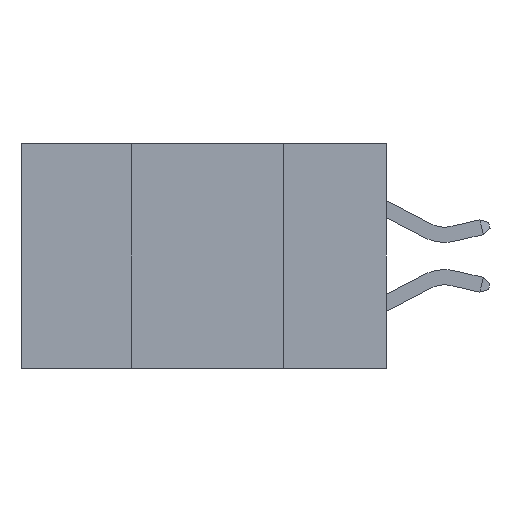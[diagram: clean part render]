
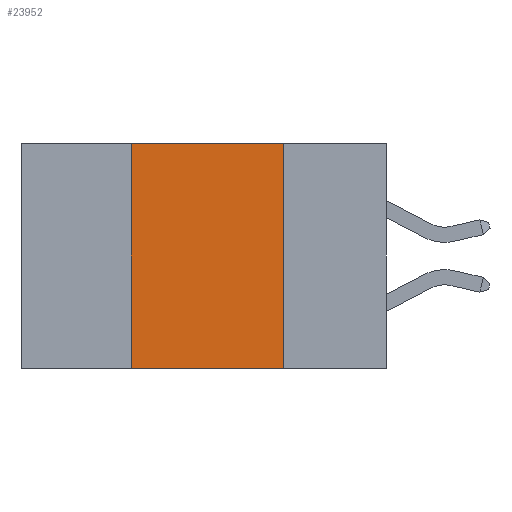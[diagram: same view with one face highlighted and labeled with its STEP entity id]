
A CAD part, left-side view. The second image highlights one B-rep face of the part: STEP entity #23952.
In plain terms, the highlighted planar face has unit normal (-1, 0, 0).
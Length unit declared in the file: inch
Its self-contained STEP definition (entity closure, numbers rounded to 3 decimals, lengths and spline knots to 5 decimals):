
#594 = LINE ( 'NONE', #15089, #6011 ) ;
#796 = VECTOR ( 'NONE', #20735, 39.37008 ) ;
#1096 = FACE_OUTER_BOUND ( 'NONE', #6258, .T. ) ;
#1642 = VERTEX_POINT ( 'NONE', #17662 ) ;
#1765 = EDGE_CURVE ( 'NONE', #1642, #24091, #3038, .T. ) ;
#2606 = EDGE_CURVE ( 'NONE', #1642, #14777, #594, .T. ) ;
#2847 = VECTOR ( 'NONE', #5439, 39.37008 ) ;
#3038 = LINE ( 'NONE', #17379, #25171 ) ;
#5439 = DIRECTION ( 'NONE',  ( 0., -1., 0. ) ) ;
#6011 = VECTOR ( 'NONE', #6787, 39.37008 ) ;
#6258 = EDGE_LOOP ( 'NONE', ( #8820, #11707, #11270, #15451 ) ) ;
#6787 = DIRECTION ( 'NONE',  ( 0., 0., 1. ) ) ;
#8058 = AXIS2_PLACEMENT_3D ( 'NONE', #13023, #9272, #19251 ) ;
#8820 = ORIENTED_EDGE ( 'NONE', *, *, #14018, .F. ) ;
#9272 = DIRECTION ( 'NONE',  ( 1., 0., 0. ) ) ;
#11270 = ORIENTED_EDGE ( 'NONE', *, *, #2606, .F. ) ;
#11707 = ORIENTED_EDGE ( 'NONE', *, *, #21804, .F. ) ;
#12501 = LINE ( 'NONE', #16564, #796 ) ;
#13023 = CARTESIAN_POINT ( 'NONE',  ( 0., 0.6, 0. ) ) ;
#14018 = EDGE_CURVE ( 'NONE', #20674, #24091, #12501, .T. ) ;
#14777 = VERTEX_POINT ( 'NONE', #15991 ) ;
#14785 = PLANE ( 'NONE',  #8058 ) ;
#15089 = CARTESIAN_POINT ( 'NONE',  ( 0., 0.42, -0.37 ) ) ;
#15451 = ORIENTED_EDGE ( 'NONE', *, *, #1765, .T. ) ;
#15886 = CARTESIAN_POINT ( 'NONE',  ( 0., 0.17, -0.37 ) ) ;
#15991 = CARTESIAN_POINT ( 'NONE',  ( 0., 0.42, 0. ) ) ;
#16320 = CARTESIAN_POINT ( 'NONE',  ( 0., 0.17, 0. ) ) ;
#16564 = CARTESIAN_POINT ( 'NONE',  ( 0., 0.17, -0.37 ) ) ;
#17379 = CARTESIAN_POINT ( 'NONE',  ( 0., 0.6, -0.37 ) ) ;
#17662 = CARTESIAN_POINT ( 'NONE',  ( 0., 0.42, -0.37 ) ) ;
#18285 = LINE ( 'NONE', #23865, #2847 ) ;
#19251 = DIRECTION ( 'NONE',  ( 0., 0., -1. ) ) ;
#20674 = VERTEX_POINT ( 'NONE', #16320 ) ;
#20735 = DIRECTION ( 'NONE',  ( 0., 0., -1. ) ) ;
#21804 = EDGE_CURVE ( 'NONE', #14777, #20674, #18285, .T. ) ;
#23865 = CARTESIAN_POINT ( 'NONE',  ( 0., 0.6, 0. ) ) ;
#23952 = ADVANCED_FACE ( 'NONE', ( #1096 ), #14785, .F. ) ;
#24091 = VERTEX_POINT ( 'NONE', #15886 ) ;
#25171 = VECTOR ( 'NONE', #25624, 39.37008 ) ;
#25624 = DIRECTION ( 'NONE',  ( 0., -1., 0. ) ) ;
